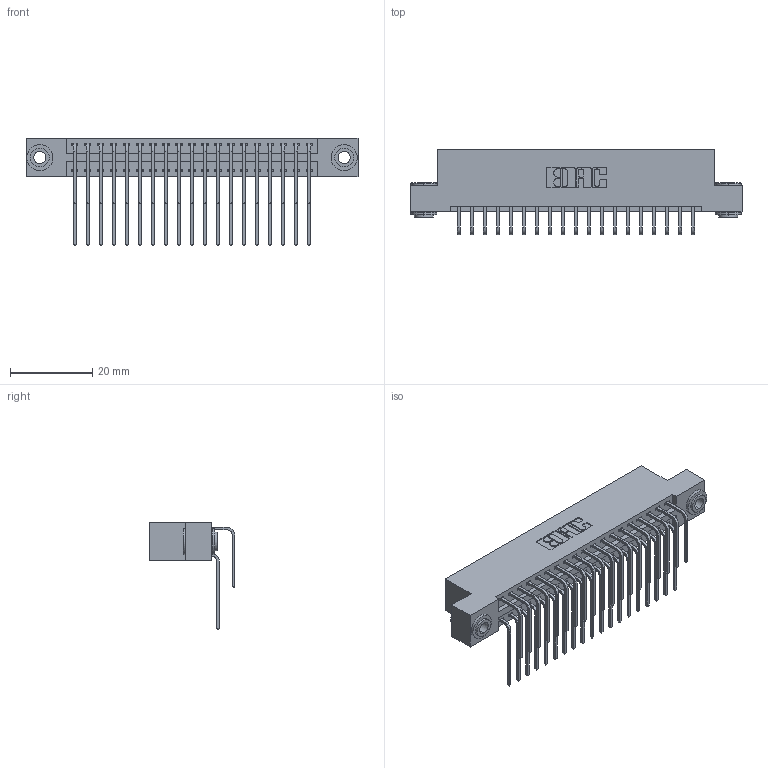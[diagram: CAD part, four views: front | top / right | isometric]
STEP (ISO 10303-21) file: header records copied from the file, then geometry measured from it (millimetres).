
FILE_DESCRIPTION (( 'STEP AP203' ), '1' );
FILE_NAME ('346-038-559-203.STEP', '2022-05-20T00:36:24', ( '' ), ( '' ), 'SwSTEP 2.0', 'SolidWorks 2020', '' );
FILE_SCHEMA (( 'CONFIG_CONTROL_DESIGN' ));
Length unit declared in the file: inch
Products named in the file (5): 345-292-001_558 559 Tail - 1; 346 Part_Flush Mounting Lugs - 0.156 Dia-TH; 346-038-559-203; 345-250-002_345-250-002-102; 345-292-001_559 Tail - 2
Assembly tree (41 placements, depth 2):
  346-038-559-203
    346 Part_Flush Mounting Lugs - 0.156 Dia-TH
    345-292-001_558 559 Tail - 1  x19
    345-292-001_559 Tail - 2  x19
    345-250-002_345-250-002-102  x2
Bounding box: 80.9 x 20.89 x 26.16 mm (x, y, z)
Volume: 7930.5 mm3; surface area: 11839.9 mm2
Topology: 41 solids, 41 shells, 2226 faces, 6559 edges, 4318 vertices
Faces by surface type: plane 1506, cylinder 712, cone 8
Entity records: 18346 total; most frequent: CARTESIAN_POINT 3088, ORIENTED_EDGE 2962, DIRECTION 2775, EDGE_CURVE 1481, LINE 1209, VECTOR 1209, VERTEX_POINT 982, AXIS2_PLACEMENT_3D 783
